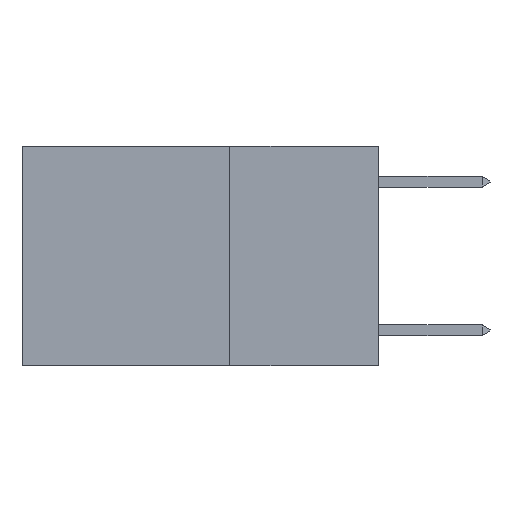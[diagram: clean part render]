
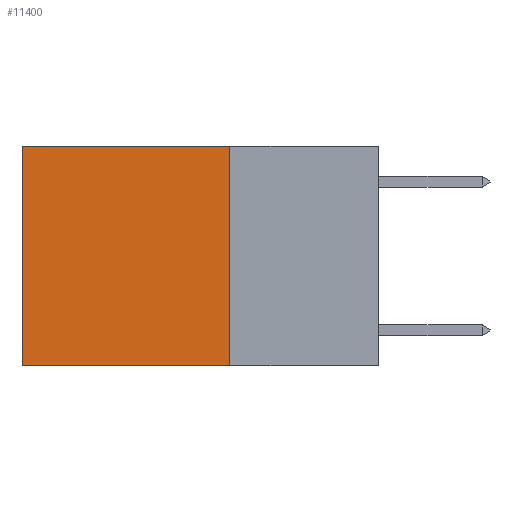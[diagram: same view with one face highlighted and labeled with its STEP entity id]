
A CAD part, left-side view. The second image highlights one B-rep face of the part: STEP entity #11400.
In plain terms, the highlighted planar face has unit normal (-1, 0, 0).
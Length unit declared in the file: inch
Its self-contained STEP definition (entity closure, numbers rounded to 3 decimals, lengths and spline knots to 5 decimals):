
#1435 = CARTESIAN_POINT ( 'NONE',  ( 0.2625, 0.25, 0. ) ) ;
#1801 = ORIENTED_EDGE ( 'NONE', *, *, #10266, .T. ) ;
#2904 = VERTEX_POINT ( 'NONE', #1435 ) ;
#3311 = DIRECTION ( 'NONE',  ( 0., 0., -1. ) ) ;
#3647 = DIRECTION ( 'NONE',  ( 0., 1., 0. ) ) ;
#3693 = EDGE_CURVE ( 'NONE', #2904, #4014, #5595, .T. ) ;
#3796 = VECTOR ( 'NONE', #5438, 39.37008 ) ;
#3910 = DIRECTION ( 'NONE',  ( 0., 1., 0. ) ) ;
#4014 = VERTEX_POINT ( 'NONE', #10557 ) ;
#4397 = CARTESIAN_POINT ( 'NONE',  ( 0.2625, 0.25, 0. ) ) ;
#5008 = VERTEX_POINT ( 'NONE', #8053 ) ;
#5217 = VECTOR ( 'NONE', #3311, 39.37008 ) ;
#5438 = DIRECTION ( 'NONE',  ( 0., 0., -1. ) ) ;
#5595 = LINE ( 'NONE', #4397, #5217 ) ;
#5711 = EDGE_CURVE ( 'NONE', #4014, #10269, #9478, .T. ) ;
#6313 = DIRECTION ( 'NONE',  ( 0., 0., -1. ) ) ;
#6576 = VECTOR ( 'NONE', #3910, 39.37008 ) ;
#7262 = PLANE ( 'NONE',  #10656 ) ;
#7624 = EDGE_CURVE ( 'NONE', #5008, #10269, #13427, .T. ) ;
#7799 = CARTESIAN_POINT ( 'NONE',  ( 0.2625, 0.6, 0. ) ) ;
#8053 = CARTESIAN_POINT ( 'NONE',  ( 0.2625, 0.6, 0. ) ) ;
#8441 = FACE_OUTER_BOUND ( 'NONE', #12788, .T. ) ;
#8745 = ORIENTED_EDGE ( 'NONE', *, *, #3693, .F. ) ;
#9212 = LINE ( 'NONE', #13691, #13217 ) ;
#9478 = LINE ( 'NONE', #13960, #6576 ) ;
#10266 = EDGE_CURVE ( 'NONE', #2904, #5008, #9212, .T. ) ;
#10269 = VERTEX_POINT ( 'NONE', #12657 ) ;
#10557 = CARTESIAN_POINT ( 'NONE',  ( 0.2625, 0.25, -0.37 ) ) ;
#10656 = AXIS2_PLACEMENT_3D ( 'NONE', #12902, #14223, #6313 ) ;
#11016 = ORIENTED_EDGE ( 'NONE', *, *, #5711, .F. ) ;
#11400 = ADVANCED_FACE ( 'NONE', ( #8441 ), #7262, .F. ) ;
#12657 = CARTESIAN_POINT ( 'NONE',  ( 0.2625, 0.6, -0.37 ) ) ;
#12788 = EDGE_LOOP ( 'NONE', ( #14073, #11016, #8745, #1801 ) ) ;
#12902 = CARTESIAN_POINT ( 'NONE',  ( 0.2625, 0.25, 0. ) ) ;
#13217 = VECTOR ( 'NONE', #3647, 39.37008 ) ;
#13427 = LINE ( 'NONE', #7799, #3796 ) ;
#13691 = CARTESIAN_POINT ( 'NONE',  ( 0.2625, 0.25, 0. ) ) ;
#13960 = CARTESIAN_POINT ( 'NONE',  ( 0.2625, 0.25, -0.37 ) ) ;
#14073 = ORIENTED_EDGE ( 'NONE', *, *, #7624, .T. ) ;
#14223 = DIRECTION ( 'NONE',  ( 1., 0., 0. ) ) ;
